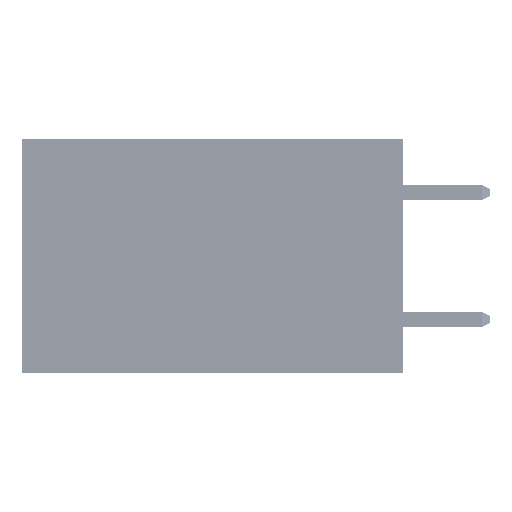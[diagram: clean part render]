
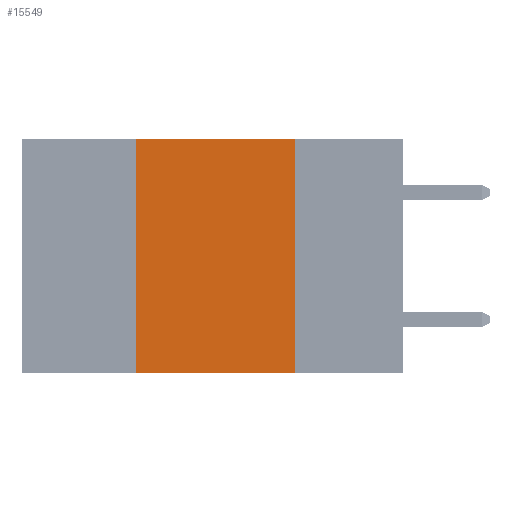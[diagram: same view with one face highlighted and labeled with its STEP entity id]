
A CAD part, left-side view. The second image highlights one B-rep face of the part: STEP entity #15549.
In plain terms, the highlighted planar face has unit normal (-1, 0, 0).
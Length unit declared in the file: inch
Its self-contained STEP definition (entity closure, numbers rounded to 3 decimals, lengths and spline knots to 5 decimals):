
#994 = CARTESIAN_POINT ( 'NONE',  ( 0., 0.17, 0. ) ) ;
#1573 = EDGE_LOOP ( 'NONE', ( #49666, #24541, #14221, #45180 ) ) ;
#2007 = DIRECTION ( 'NONE',  ( 0., 0., 1. ) ) ;
#2331 = CARTESIAN_POINT ( 'NONE',  ( 0., 0.42, 0. ) ) ;
#5098 = CARTESIAN_POINT ( 'NONE',  ( 0., 0.6, 0. ) ) ;
#8800 = LINE ( 'NONE', #17802, #38353 ) ;
#9800 = VERTEX_POINT ( 'NONE', #49399 ) ;
#11619 = VECTOR ( 'NONE', #2007, 39.37008 ) ;
#12284 = LINE ( 'NONE', #47547, #34010 ) ;
#14221 = ORIENTED_EDGE ( 'NONE', *, *, #42646, .F. ) ;
#15549 = ADVANCED_FACE ( 'NONE', ( #49425 ), #46203, .F. ) ;
#17802 = CARTESIAN_POINT ( 'NONE',  ( 0., 0.17, 0. ) ) ;
#18309 = DIRECTION ( 'NONE',  ( 0., 0., -1. ) ) ;
#20586 = DIRECTION ( 'NONE',  ( 0., -1., 0. ) ) ;
#23105 = DIRECTION ( 'NONE',  ( 1., 0., 0. ) ) ;
#24287 = AXIS2_PLACEMENT_3D ( 'NONE', #5098, #23105, #24310 ) ;
#24310 = DIRECTION ( 'NONE',  ( 0., 0., -1. ) ) ;
#24541 = ORIENTED_EDGE ( 'NONE', *, *, #27077, .F. ) ;
#27077 = EDGE_CURVE ( 'NONE', #9800, #33358, #29006, .T. ) ;
#27300 = LINE ( 'NONE', #2331, #11619 ) ;
#29006 = LINE ( 'NONE', #31895, #43398 ) ;
#31895 = CARTESIAN_POINT ( 'NONE',  ( 0., 0.6, 0. ) ) ;
#33358 = VERTEX_POINT ( 'NONE', #994 ) ;
#34010 = VECTOR ( 'NONE', #20586, 39.37008 ) ;
#35746 = DIRECTION ( 'NONE',  ( 0., -1., 0. ) ) ;
#38353 = VECTOR ( 'NONE', #18309, 39.37008 ) ;
#39754 = VERTEX_POINT ( 'NONE', #39889 ) ;
#39889 = CARTESIAN_POINT ( 'NONE',  ( 0., 0.17, -0.37 ) ) ;
#40725 = EDGE_CURVE ( 'NONE', #33358, #39754, #8800, .T. ) ;
#41762 = EDGE_CURVE ( 'NONE', #48506, #39754, #12284, .T. ) ;
#42646 = EDGE_CURVE ( 'NONE', #48506, #9800, #27300, .T. ) ;
#43398 = VECTOR ( 'NONE', #35746, 39.37008 ) ;
#45180 = ORIENTED_EDGE ( 'NONE', *, *, #41762, .T. ) ;
#46203 = PLANE ( 'NONE',  #24287 ) ;
#46657 = CARTESIAN_POINT ( 'NONE',  ( 0., 0.42, -0.37 ) ) ;
#47547 = CARTESIAN_POINT ( 'NONE',  ( 0., 0.6, -0.37 ) ) ;
#48506 = VERTEX_POINT ( 'NONE', #46657 ) ;
#49399 = CARTESIAN_POINT ( 'NONE',  ( 0., 0.42, 0. ) ) ;
#49425 = FACE_OUTER_BOUND ( 'NONE', #1573, .T. ) ;
#49666 = ORIENTED_EDGE ( 'NONE', *, *, #40725, .F. ) ;
